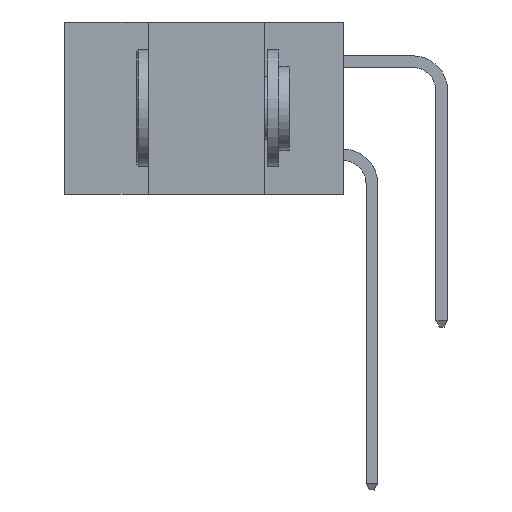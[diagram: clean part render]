
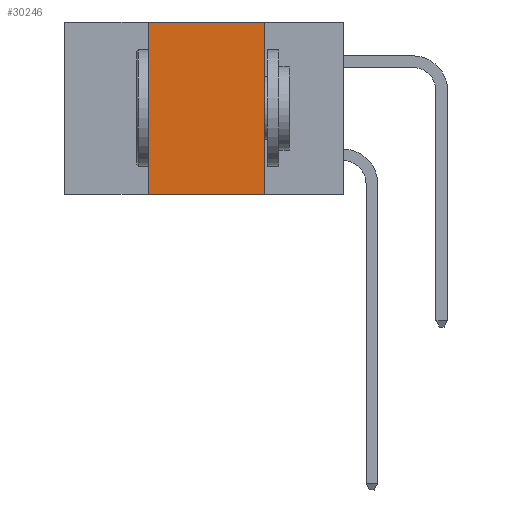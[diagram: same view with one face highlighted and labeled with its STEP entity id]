
A CAD part, left-side view. The second image highlights one B-rep face of the part: STEP entity #30246.
In plain terms, the highlighted planar face has unit normal (-1, 0, 0).
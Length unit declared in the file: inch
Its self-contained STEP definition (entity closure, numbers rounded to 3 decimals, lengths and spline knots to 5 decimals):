
#62 = DIRECTION ( 'NONE',  ( 0., 0., -1. ) ) ;
#847 = VECTOR ( 'NONE', #62, 39.37008 ) ;
#2014 = DIRECTION ( 'NONE',  ( 0., 0., 1. ) ) ;
#4098 = ORIENTED_EDGE ( 'NONE', *, *, #15071, .F. ) ;
#4362 = AXIS2_PLACEMENT_3D ( 'NONE', #19444, #4985, #21845 ) ;
#4985 = DIRECTION ( 'NONE',  ( 1., 0., 0. ) ) ;
#5799 = VECTOR ( 'NONE', #19386, 39.37008 ) ;
#5906 = VECTOR ( 'NONE', #27119, 39.37008 ) ;
#7337 = VERTEX_POINT ( 'NONE', #7894 ) ;
#7635 = CARTESIAN_POINT ( 'NONE',  ( 0., 0.42, 0. ) ) ;
#7894 = CARTESIAN_POINT ( 'NONE',  ( 0., 0.17, -0.37 ) ) ;
#8088 = LINE ( 'NONE', #24131, #847 ) ;
#8596 = LINE ( 'NONE', #30945, #27123 ) ;
#11835 = ORIENTED_EDGE ( 'NONE', *, *, #28193, .T. ) ;
#11851 = VERTEX_POINT ( 'NONE', #21234 ) ;
#12163 = PLANE ( 'NONE',  #4362 ) ;
#12631 = EDGE_CURVE ( 'NONE', #11851, #7337, #8088, .T. ) ;
#15071 = EDGE_CURVE ( 'NONE', #20916, #11851, #18654, .T. ) ;
#16968 = CARTESIAN_POINT ( 'NONE',  ( 0., 0.6, 0. ) ) ;
#18654 = LINE ( 'NONE', #16968, #5799 ) ;
#18757 = LINE ( 'NONE', #24671, #5906 ) ;
#19386 = DIRECTION ( 'NONE',  ( 0., -1., 0. ) ) ;
#19444 = CARTESIAN_POINT ( 'NONE',  ( 0., 0.6, 0. ) ) ;
#20712 = EDGE_CURVE ( 'NONE', #27737, #20916, #8596, .T. ) ;
#20916 = VERTEX_POINT ( 'NONE', #7635 ) ;
#21234 = CARTESIAN_POINT ( 'NONE',  ( 0., 0.17, 0. ) ) ;
#21519 = EDGE_LOOP ( 'NONE', ( #28252, #4098, #29849, #11835 ) ) ;
#21845 = DIRECTION ( 'NONE',  ( 0., 0., -1. ) ) ;
#24131 = CARTESIAN_POINT ( 'NONE',  ( 0., 0.17, 0. ) ) ;
#24671 = CARTESIAN_POINT ( 'NONE',  ( 0., 0.6, -0.37 ) ) ;
#27119 = DIRECTION ( 'NONE',  ( 0., -1., 0. ) ) ;
#27123 = VECTOR ( 'NONE', #2014, 39.37008 ) ;
#27239 = CARTESIAN_POINT ( 'NONE',  ( 0., 0.42, -0.37 ) ) ;
#27737 = VERTEX_POINT ( 'NONE', #27239 ) ;
#28193 = EDGE_CURVE ( 'NONE', #27737, #7337, #18757, .T. ) ;
#28252 = ORIENTED_EDGE ( 'NONE', *, *, #12631, .F. ) ;
#29849 = ORIENTED_EDGE ( 'NONE', *, *, #20712, .F. ) ;
#29988 = FACE_OUTER_BOUND ( 'NONE', #21519, .T. ) ;
#30246 = ADVANCED_FACE ( 'NONE', ( #29988 ), #12163, .F. ) ;
#30945 = CARTESIAN_POINT ( 'NONE',  ( 0., 0.42, 0. ) ) ;
